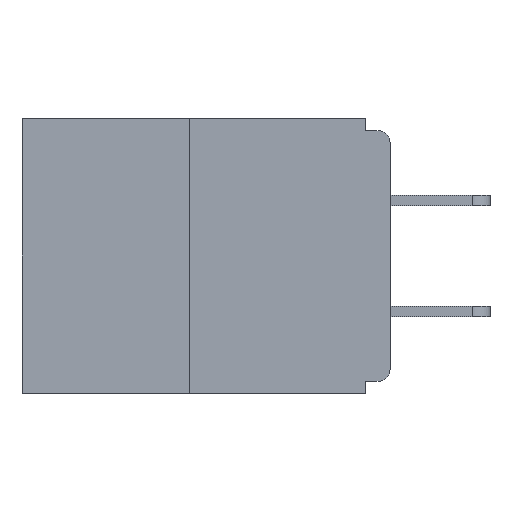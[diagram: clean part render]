
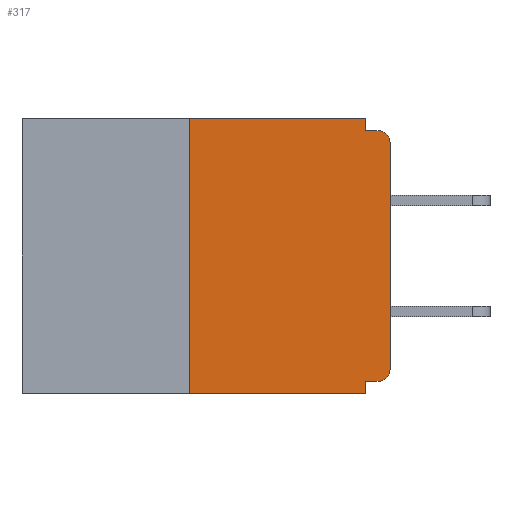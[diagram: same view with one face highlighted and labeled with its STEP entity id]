
A CAD part, left-side view. The second image highlights one B-rep face of the part: STEP entity #317.
In plain terms, the highlighted planar face has unit normal (-1, 0, 0).
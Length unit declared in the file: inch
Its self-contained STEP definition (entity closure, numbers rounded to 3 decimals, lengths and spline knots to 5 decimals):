
#317 = ADVANCED_FACE ( 'NONE', ( #4871 ), #4763, .F. ) ;
#445 = CARTESIAN_POINT ( 'NONE',  ( 0., 0.46, 0. ) ) ;
#510 = VECTOR ( 'NONE', #7391, 39.37008 ) ;
#559 = CARTESIAN_POINT ( 'NONE',  ( 0., 0., -0.015 ) ) ;
#600 = DIRECTION ( 'NONE',  ( 0., -1., 0. ) ) ;
#655 = CARTESIAN_POINT ( 'NONE',  ( 0., 0.031, -0.015 ) ) ;
#731 = DIRECTION ( 'NONE',  ( 0., 0., -1. ) ) ;
#1148 = VECTOR ( 'NONE', #731, 39.37008 ) ;
#1203 = DIRECTION ( 'NONE',  ( 0., 0., 1. ) ) ;
#1251 = LINE ( 'NONE', #4916, #2746 ) ;
#1269 = EDGE_CURVE ( 'NONE', #10436, #4632, #9146, .T. ) ;
#1384 = LINE ( 'NONE', #9482, #6253 ) ;
#1438 = AXIS2_PLACEMENT_3D ( 'NONE', #7766, #5248, #6033 ) ;
#1451 = VERTEX_POINT ( 'NONE', #7882 ) ;
#1527 = CARTESIAN_POINT ( 'NONE',  ( 0., 0.031, 0. ) ) ;
#1731 = CARTESIAN_POINT ( 'NONE',  ( 0., 0., -0.03 ) ) ;
#1760 = CARTESIAN_POINT ( 'NONE',  ( 0., 0.25, -0.343 ) ) ;
#2441 = DIRECTION ( 'NONE',  ( -1., 0., 0. ) ) ;
#2536 = VERTEX_POINT ( 'NONE', #10045 ) ;
#2746 = VECTOR ( 'NONE', #8180, 39.37008 ) ;
#2879 = EDGE_CURVE ( 'NONE', #8871, #10436, #1384, .T. ) ;
#3297 = CARTESIAN_POINT ( 'NONE',  ( 0., 0.031, -0.343 ) ) ;
#3821 = ORIENTED_EDGE ( 'NONE', *, *, #9050, .F. ) ;
#3863 = ORIENTED_EDGE ( 'NONE', *, *, #1269, .T. ) ;
#4222 = DIRECTION ( 'NONE',  ( 0., 0., -1. ) ) ;
#4365 = VERTEX_POINT ( 'NONE', #9389 ) ;
#4632 = VERTEX_POINT ( 'NONE', #7508 ) ;
#4639 = DIRECTION ( 'NONE',  ( 0., -1., 0. ) ) ;
#4688 = VECTOR ( 'NONE', #4639, 39.37008 ) ;
#4763 = PLANE ( 'NONE',  #11096 ) ;
#4871 = FACE_OUTER_BOUND ( 'NONE', #9995, .T. ) ;
#4916 = CARTESIAN_POINT ( 'NONE',  ( 0., 0.46, -0.343 ) ) ;
#5131 = LINE ( 'NONE', #10855, #510 ) ;
#5135 = CARTESIAN_POINT ( 'NONE',  ( 0., 0., -0.328 ) ) ;
#5170 = DIRECTION ( 'NONE',  ( 0., 1., 0. ) ) ;
#5238 = VERTEX_POINT ( 'NONE', #7009 ) ;
#5248 = DIRECTION ( 'NONE',  ( -1., 0., 0. ) ) ;
#5345 = AXIS2_PLACEMENT_3D ( 'NONE', #9369, #2441, #4222 ) ;
#5526 = ORIENTED_EDGE ( 'NONE', *, *, #11081, .F. ) ;
#5807 = DIRECTION ( 'NONE',  ( 0., 0., -1. ) ) ;
#5905 = EDGE_CURVE ( 'NONE', #6719, #2536, #7863, .T. ) ;
#6033 = DIRECTION ( 'NONE',  ( 0., 0., -1. ) ) ;
#6131 = VECTOR ( 'NONE', #600, 39.37008 ) ;
#6162 = VECTOR ( 'NONE', #5170, 39.37008 ) ;
#6253 = VECTOR ( 'NONE', #10339, 39.37008 ) ;
#6382 = LINE ( 'NONE', #559, #6131 ) ;
#6409 = EDGE_CURVE ( 'NONE', #8964, #4632, #6382, .T. ) ;
#6460 = EDGE_CURVE ( 'NONE', #6719, #10322, #1251, .T. ) ;
#6474 = DIRECTION ( 'NONE',  ( 1., 0., 0. ) ) ;
#6719 = VERTEX_POINT ( 'NONE', #1760 ) ;
#6739 = CIRCLE ( 'NONE', #1438, 0.015 ) ;
#6957 = ORIENTED_EDGE ( 'NONE', *, *, #8497, .T. ) ;
#7009 = CARTESIAN_POINT ( 'NONE',  ( 0., 0.031, -0.328 ) ) ;
#7327 = CARTESIAN_POINT ( 'NONE',  ( 0., 0., -0.313 ) ) ;
#7391 = DIRECTION ( 'NONE',  ( 0., 0., -1. ) ) ;
#7508 = CARTESIAN_POINT ( 'NONE',  ( 0., 0.015, -0.015 ) ) ;
#7586 = VECTOR ( 'NONE', #1203, 39.37008 ) ;
#7766 = CARTESIAN_POINT ( 'NONE',  ( 0., 0.015, -0.313 ) ) ;
#7775 = LINE ( 'NONE', #5135, #6162 ) ;
#7863 = LINE ( 'NONE', #8979, #7586 ) ;
#7882 = CARTESIAN_POINT ( 'NONE',  ( 0., 0.015, -0.328 ) ) ;
#8031 = LINE ( 'NONE', #8702, #4688 ) ;
#8059 = ORIENTED_EDGE ( 'NONE', *, *, #6460, .T. ) ;
#8180 = DIRECTION ( 'NONE',  ( 0., -1., 0. ) ) ;
#8497 = EDGE_CURVE ( 'NONE', #1451, #8871, #6739, .T. ) ;
#8702 = CARTESIAN_POINT ( 'NONE',  ( 0., 0.46, 0. ) ) ;
#8871 = VERTEX_POINT ( 'NONE', #7327 ) ;
#8964 = VERTEX_POINT ( 'NONE', #655 ) ;
#8979 = CARTESIAN_POINT ( 'NONE',  ( 0., 0.25, 0. ) ) ;
#9050 = EDGE_CURVE ( 'NONE', #5238, #10322, #5131, .T. ) ;
#9146 = CIRCLE ( 'NONE', #5345, 0.015 ) ;
#9337 = ORIENTED_EDGE ( 'NONE', *, *, #6409, .F. ) ;
#9369 = CARTESIAN_POINT ( 'NONE',  ( 0., 0.015, -0.03 ) ) ;
#9389 = CARTESIAN_POINT ( 'NONE',  ( 0., 0.031, 0. ) ) ;
#9482 = CARTESIAN_POINT ( 'NONE',  ( 0., 0., 0. ) ) ;
#9529 = ORIENTED_EDGE ( 'NONE', *, *, #2879, .T. ) ;
#9995 = EDGE_LOOP ( 'NONE', ( #10182, #10411, #8059, #3821, #10563, #6957, #9529, #3863, #9337, #5526 ) ) ;
#10045 = CARTESIAN_POINT ( 'NONE',  ( 0., 0.25, 0. ) ) ;
#10182 = ORIENTED_EDGE ( 'NONE', *, *, #10599, .F. ) ;
#10322 = VERTEX_POINT ( 'NONE', #3297 ) ;
#10339 = DIRECTION ( 'NONE',  ( 0., 0., 1. ) ) ;
#10411 = ORIENTED_EDGE ( 'NONE', *, *, #5905, .F. ) ;
#10424 = EDGE_CURVE ( 'NONE', #1451, #5238, #7775, .T. ) ;
#10436 = VERTEX_POINT ( 'NONE', #1731 ) ;
#10563 = ORIENTED_EDGE ( 'NONE', *, *, #10424, .F. ) ;
#10599 = EDGE_CURVE ( 'NONE', #2536, #4365, #8031, .T. ) ;
#10601 = LINE ( 'NONE', #1527, #1148 ) ;
#10855 = CARTESIAN_POINT ( 'NONE',  ( 0., 0.031, -0.343 ) ) ;
#11081 = EDGE_CURVE ( 'NONE', #4365, #8964, #10601, .T. ) ;
#11096 = AXIS2_PLACEMENT_3D ( 'NONE', #445, #6474, #5807 ) ;
